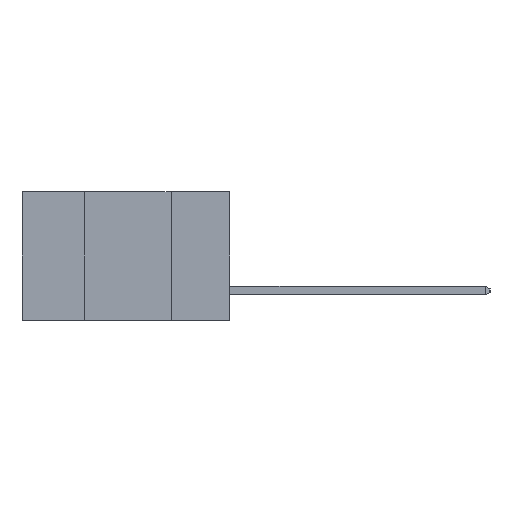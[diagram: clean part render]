
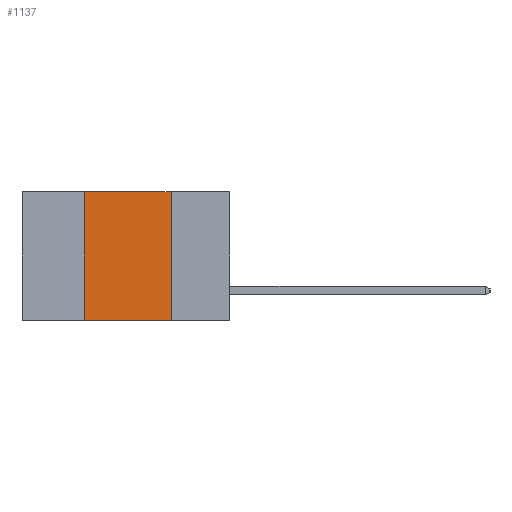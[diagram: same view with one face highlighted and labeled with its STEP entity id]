
A CAD part, left-side view. The second image highlights one B-rep face of the part: STEP entity #1137.
In plain terms, the highlighted planar face has unit normal (-1, 0, 0).
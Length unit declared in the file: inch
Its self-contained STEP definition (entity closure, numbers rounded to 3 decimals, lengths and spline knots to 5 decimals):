
#57 = CARTESIAN_POINT ( 'NONE',  ( 0., 0.42, 0. ) ) ;
#187 = CARTESIAN_POINT ( 'NONE',  ( 0., 0.17, -0.37 ) ) ;
#279 = EDGE_CURVE ( 'NONE', #9884, #665, #8198, .T. ) ;
#543 = VECTOR ( 'NONE', #8979, 39.37008 ) ;
#587 = VECTOR ( 'NONE', #11624, 39.37008 ) ;
#665 = VERTEX_POINT ( 'NONE', #187 ) ;
#910 = DIRECTION ( 'NONE',  ( 1., 0., 0. ) ) ;
#1038 = VECTOR ( 'NONE', #5861, 39.37008 ) ;
#1062 = ORIENTED_EDGE ( 'NONE', *, *, #4067, .T. ) ;
#1137 = ADVANCED_FACE ( 'NONE', ( #4111 ), #11197, .F. ) ;
#3168 = CARTESIAN_POINT ( 'NONE',  ( 0., 0.42, -0.37 ) ) ;
#3485 = LINE ( 'NONE', #10759, #543 ) ;
#3644 = LINE ( 'NONE', #57, #1038 ) ;
#4067 = EDGE_CURVE ( 'NONE', #9465, #665, #7114, .T. ) ;
#4111 = FACE_OUTER_BOUND ( 'NONE', #9287, .T. ) ;
#5004 = ORIENTED_EDGE ( 'NONE', *, *, #279, .F. ) ;
#5464 = ORIENTED_EDGE ( 'NONE', *, *, #8433, .F. ) ;
#5646 = CARTESIAN_POINT ( 'NONE',  ( 0., 0.42, 0. ) ) ;
#5861 = DIRECTION ( 'NONE',  ( 0., 0., 1. ) ) ;
#6551 = CARTESIAN_POINT ( 'NONE',  ( 0., 0.17, 0. ) ) ;
#6677 = CARTESIAN_POINT ( 'NONE',  ( 0., 0.6, 0. ) ) ;
#7114 = LINE ( 'NONE', #9122, #11636 ) ;
#7128 = AXIS2_PLACEMENT_3D ( 'NONE', #6677, #910, #7603 ) ;
#7514 = ORIENTED_EDGE ( 'NONE', *, *, #8193, .F. ) ;
#7603 = DIRECTION ( 'NONE',  ( 0., 0., -1. ) ) ;
#8193 = EDGE_CURVE ( 'NONE', #9465, #9900, #3644, .T. ) ;
#8198 = LINE ( 'NONE', #10696, #587 ) ;
#8433 = EDGE_CURVE ( 'NONE', #9900, #9884, #3485, .T. ) ;
#8979 = DIRECTION ( 'NONE',  ( 0., -1., 0. ) ) ;
#9122 = CARTESIAN_POINT ( 'NONE',  ( 0., 0.6, -0.37 ) ) ;
#9287 = EDGE_LOOP ( 'NONE', ( #5004, #5464, #7514, #1062 ) ) ;
#9465 = VERTEX_POINT ( 'NONE', #3168 ) ;
#9884 = VERTEX_POINT ( 'NONE', #6551 ) ;
#9900 = VERTEX_POINT ( 'NONE', #5646 ) ;
#10028 = DIRECTION ( 'NONE',  ( 0., -1., 0. ) ) ;
#10696 = CARTESIAN_POINT ( 'NONE',  ( 0., 0.17, 0. ) ) ;
#10759 = CARTESIAN_POINT ( 'NONE',  ( 0., 0.6, 0. ) ) ;
#11197 = PLANE ( 'NONE',  #7128 ) ;
#11624 = DIRECTION ( 'NONE',  ( 0., 0., -1. ) ) ;
#11636 = VECTOR ( 'NONE', #10028, 39.37008 ) ;
